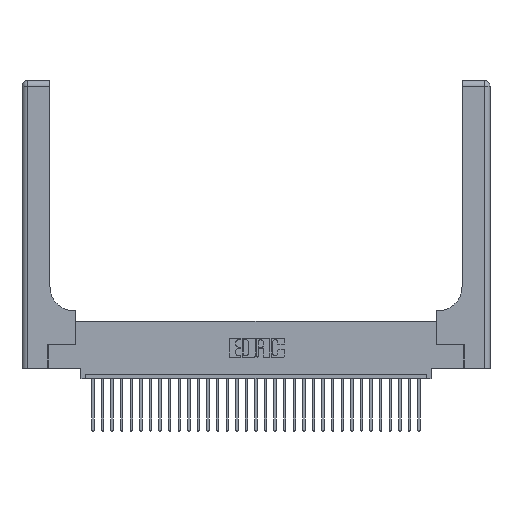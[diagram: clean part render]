
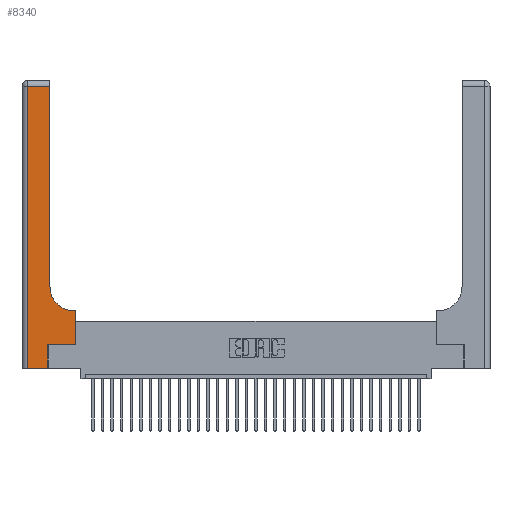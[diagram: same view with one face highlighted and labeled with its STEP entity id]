
A CAD part, top view. The second image highlights one B-rep face of the part: STEP entity #8340.
In plain terms, the highlighted planar face has unit normal (0, 0, 1).
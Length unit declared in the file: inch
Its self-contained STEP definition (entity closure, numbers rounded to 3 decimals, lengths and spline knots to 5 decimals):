
#694 = CARTESIAN_POINT ( 'NONE',  ( 0.2915, 2.94, 0.37 ) ) ;
#1048 = EDGE_LOOP ( 'NONE', ( #25019, #18760, #14087, #26884, #18976, #21767, #29225, #13909, #19128 ) ) ;
#1988 = EDGE_CURVE ( 'NONE', #27646, #29488, #17047, .T. ) ;
#2852 = VECTOR ( 'NONE', #32179, 39.37008 ) ;
#3017 = DIRECTION ( 'NONE',  ( -1., 0., 0. ) ) ;
#3066 = VERTEX_POINT ( 'NONE', #26990 ) ;
#3307 = EDGE_CURVE ( 'NONE', #3066, #22564, #12577, .T. ) ;
#3861 = LINE ( 'NONE', #16910, #24010 ) ;
#3963 = CARTESIAN_POINT ( 'NONE',  ( 0.269, 0., 0.37 ) ) ;
#4125 = PLANE ( 'NONE',  #32416 ) ;
#4469 = VERTEX_POINT ( 'NONE', #9989 ) ;
#4662 = CARTESIAN_POINT ( 'NONE',  ( 0.2915, 3., 0.37 ) ) ;
#6092 = DIRECTION ( 'NONE',  ( 0., 1., 0. ) ) ;
#6376 = EDGE_CURVE ( 'NONE', #4469, #17932, #24565, .T. ) ;
#7006 = DIRECTION ( 'NONE',  ( 0., 0., -1. ) ) ;
#8340 = ADVANCED_FACE ( 'NONE', ( #31499 ), #4125, .F. ) ;
#8718 = DIRECTION ( 'NONE',  ( -1., 0., 0. ) ) ;
#8868 = CARTESIAN_POINT ( 'NONE',  ( 0.5585, 0.6, 0.37 ) ) ;
#9409 = VERTEX_POINT ( 'NONE', #13227 ) ;
#9989 = CARTESIAN_POINT ( 'NONE',  ( 0.5585, 0.25, 0.37 ) ) ;
#10482 = AXIS2_PLACEMENT_3D ( 'NONE', #31853, #7006, #29601 ) ;
#10595 = LINE ( 'NONE', #18310, #13360 ) ;
#11025 = VECTOR ( 'NONE', #6092, 39.37008 ) ;
#11354 = DIRECTION ( 'NONE',  ( 0., 0., -1. ) ) ;
#11825 = DIRECTION ( 'NONE',  ( 1., 0., 0. ) ) ;
#12577 = LINE ( 'NONE', #4662, #30383 ) ;
#13227 = CARTESIAN_POINT ( 'NONE',  ( 0.5415, 0.6, 0.37 ) ) ;
#13360 = VECTOR ( 'NONE', #3017, 39.37008 ) ;
#13909 = ORIENTED_EDGE ( 'NONE', *, *, #21740, .T. ) ;
#14087 = ORIENTED_EDGE ( 'NONE', *, *, #28568, .T. ) ;
#14498 = CARTESIAN_POINT ( 'NONE',  ( 0.269, 0., 0.37 ) ) ;
#14592 = LINE ( 'NONE', #18682, #32360 ) ;
#16910 = CARTESIAN_POINT ( 'NONE',  ( 0.269, 0.25, 0.37 ) ) ;
#17047 = LINE ( 'NONE', #14498, #2852 ) ;
#17472 = EDGE_CURVE ( 'NONE', #29488, #4469, #3861, .T. ) ;
#17782 = VERTEX_POINT ( 'NONE', #18884 ) ;
#17932 = VERTEX_POINT ( 'NONE', #8868 ) ;
#18086 = DIRECTION ( 'NONE',  ( 1., 0., 0. ) ) ;
#18310 = CARTESIAN_POINT ( 'NONE',  ( 0., 2.94, 0.37 ) ) ;
#18682 = CARTESIAN_POINT ( 'NONE',  ( 0.2915, 0.6, 0.37 ) ) ;
#18754 = VECTOR ( 'NONE', #18086, 39.37008 ) ;
#18760 = ORIENTED_EDGE ( 'NONE', *, *, #26477, .T. ) ;
#18884 = CARTESIAN_POINT ( 'NONE',  ( 0.06, 2.94, 0.37 ) ) ;
#18976 = ORIENTED_EDGE ( 'NONE', *, *, #1988, .T. ) ;
#19128 = ORIENTED_EDGE ( 'NONE', *, *, #24871, .T. ) ;
#19941 = LINE ( 'NONE', #30084, #18754 ) ;
#21740 = EDGE_CURVE ( 'NONE', #17932, #9409, #14592, .T. ) ;
#21767 = ORIENTED_EDGE ( 'NONE', *, *, #17472, .T. ) ;
#22564 = VERTEX_POINT ( 'NONE', #694 ) ;
#23889 = CARTESIAN_POINT ( 'NONE',  ( 0., 3., 0.37 ) ) ;
#24010 = VECTOR ( 'NONE', #11825, 39.37008 ) ;
#24543 = CARTESIAN_POINT ( 'NONE',  ( 0.06, 3., 0.37 ) ) ;
#24565 = LINE ( 'NONE', #31349, #11025 ) ;
#24871 = EDGE_CURVE ( 'NONE', #9409, #3066, #27359, .T. ) ;
#25019 = ORIENTED_EDGE ( 'NONE', *, *, #3307, .T. ) ;
#25546 = VECTOR ( 'NONE', #29616, 39.37008 ) ;
#25669 = CARTESIAN_POINT ( 'NONE',  ( 0.269, 0.25, 0.37 ) ) ;
#26350 = VERTEX_POINT ( 'NONE', #27901 ) ;
#26477 = EDGE_CURVE ( 'NONE', #22564, #17782, #10595, .T. ) ;
#26705 = DIRECTION ( 'NONE',  ( -1., 0., 0. ) ) ;
#26884 = ORIENTED_EDGE ( 'NONE', *, *, #29414, .T. ) ;
#26990 = CARTESIAN_POINT ( 'NONE',  ( 0.2915, 0.85, 0.37 ) ) ;
#27359 = CIRCLE ( 'NONE', #10482, 0.25 ) ;
#27441 = DIRECTION ( 'NONE',  ( 0., 1., 0. ) ) ;
#27646 = VERTEX_POINT ( 'NONE', #3963 ) ;
#27901 = CARTESIAN_POINT ( 'NONE',  ( 0.06, 0., 0.37 ) ) ;
#28568 = EDGE_CURVE ( 'NONE', #17782, #26350, #30281, .T. ) ;
#29225 = ORIENTED_EDGE ( 'NONE', *, *, #6376, .T. ) ;
#29414 = EDGE_CURVE ( 'NONE', #26350, #27646, #19941, .T. ) ;
#29488 = VERTEX_POINT ( 'NONE', #25669 ) ;
#29601 = DIRECTION ( 'NONE',  ( 1., 0., 0. ) ) ;
#29616 = DIRECTION ( 'NONE',  ( 0., -1., 0. ) ) ;
#30084 = CARTESIAN_POINT ( 'NONE',  ( 0., 0., 0.37 ) ) ;
#30281 = LINE ( 'NONE', #24543, #25546 ) ;
#30383 = VECTOR ( 'NONE', #27441, 39.37008 ) ;
#31349 = CARTESIAN_POINT ( 'NONE',  ( 0.5585, 0.25, 0.37 ) ) ;
#31499 = FACE_OUTER_BOUND ( 'NONE', #1048, .T. ) ;
#31853 = CARTESIAN_POINT ( 'NONE',  ( 0.5415, 0.85, 0.37 ) ) ;
#32179 = DIRECTION ( 'NONE',  ( 0., 1., 0. ) ) ;
#32360 = VECTOR ( 'NONE', #26705, 39.37008 ) ;
#32416 = AXIS2_PLACEMENT_3D ( 'NONE', #23889, #11354, #8718 ) ;
